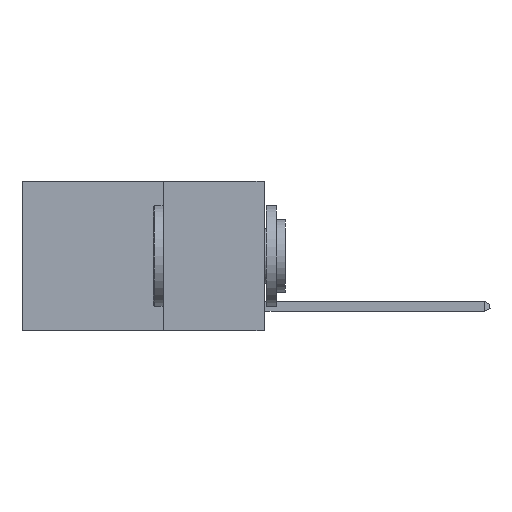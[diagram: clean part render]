
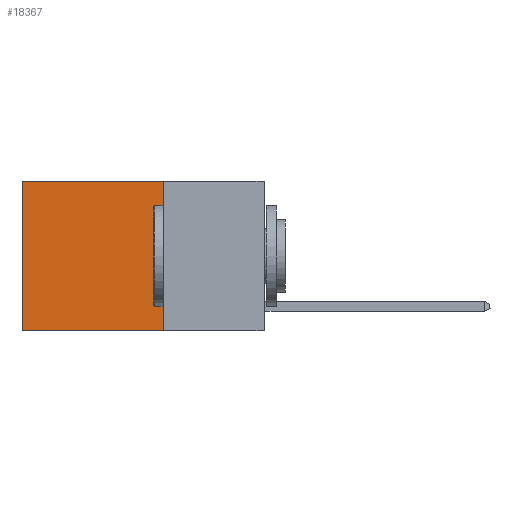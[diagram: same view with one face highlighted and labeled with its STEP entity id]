
A CAD part, left-side view. The second image highlights one B-rep face of the part: STEP entity #18367.
In plain terms, the highlighted planar face has unit normal (-1, 0, 0).
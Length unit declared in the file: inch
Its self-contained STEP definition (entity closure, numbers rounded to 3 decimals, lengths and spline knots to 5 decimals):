
#593 = EDGE_CURVE ( 'NONE', #977, #14643, #2071, .T. ) ;
#977 = VERTEX_POINT ( 'NONE', #10305 ) ;
#1006 = CARTESIAN_POINT ( 'NONE',  ( 0.2625, 0.25, 0. ) ) ;
#1887 = PLANE ( 'NONE',  #9312 ) ;
#2071 = LINE ( 'NONE', #2968, #14374 ) ;
#2121 = CARTESIAN_POINT ( 'NONE',  ( 0.2625, 0.25, -0.37 ) ) ;
#2166 = EDGE_LOOP ( 'NONE', ( #13786, #14681, #14840, #5429 ) ) ;
#2567 = CARTESIAN_POINT ( 'NONE',  ( 0.2625, 0.6, 0. ) ) ;
#2948 = DIRECTION ( 'NONE',  ( 0., 1., 0. ) ) ;
#2968 = CARTESIAN_POINT ( 'NONE',  ( 0.2625, 0.25, 0. ) ) ;
#3455 = DIRECTION ( 'NONE',  ( 1., 0., 0. ) ) ;
#3872 = CARTESIAN_POINT ( 'NONE',  ( 0.2625, 0.25, -0.37 ) ) ;
#4131 = DIRECTION ( 'NONE',  ( 0., 0., -1. ) ) ;
#5429 = ORIENTED_EDGE ( 'NONE', *, *, #593, .T. ) ;
#5892 = VECTOR ( 'NONE', #18093, 39.37008 ) ;
#7064 = VECTOR ( 'NONE', #11656, 39.37008 ) ;
#8236 = LINE ( 'NONE', #2567, #19869 ) ;
#9312 = AXIS2_PLACEMENT_3D ( 'NONE', #12699, #3455, #14236 ) ;
#10305 = CARTESIAN_POINT ( 'NONE',  ( 0.2625, 0.25, 0. ) ) ;
#10583 = EDGE_CURVE ( 'NONE', #11774, #12818, #15237, .T. ) ;
#10808 = CARTESIAN_POINT ( 'NONE',  ( 0.2625, 0.6, -0.37 ) ) ;
#11656 = DIRECTION ( 'NONE',  ( 0., 1., 0. ) ) ;
#11774 = VERTEX_POINT ( 'NONE', #2121 ) ;
#12058 = EDGE_CURVE ( 'NONE', #977, #11774, #18107, .T. ) ;
#12699 = CARTESIAN_POINT ( 'NONE',  ( 0.2625, 0.25, 0. ) ) ;
#12818 = VERTEX_POINT ( 'NONE', #10808 ) ;
#13786 = ORIENTED_EDGE ( 'NONE', *, *, #14202, .T. ) ;
#14202 = EDGE_CURVE ( 'NONE', #14643, #12818, #8236, .T. ) ;
#14236 = DIRECTION ( 'NONE',  ( 0., 0., -1. ) ) ;
#14374 = VECTOR ( 'NONE', #2948, 39.37008 ) ;
#14643 = VERTEX_POINT ( 'NONE', #18927 ) ;
#14681 = ORIENTED_EDGE ( 'NONE', *, *, #10583, .F. ) ;
#14840 = ORIENTED_EDGE ( 'NONE', *, *, #12058, .F. ) ;
#15237 = LINE ( 'NONE', #3872, #7064 ) ;
#17416 = FACE_OUTER_BOUND ( 'NONE', #2166, .T. ) ;
#18093 = DIRECTION ( 'NONE',  ( 0., 0., -1. ) ) ;
#18107 = LINE ( 'NONE', #1006, #5892 ) ;
#18367 = ADVANCED_FACE ( 'NONE', ( #17416 ), #1887, .F. ) ;
#18927 = CARTESIAN_POINT ( 'NONE',  ( 0.2625, 0.6, 0. ) ) ;
#19869 = VECTOR ( 'NONE', #4131, 39.37008 ) ;
